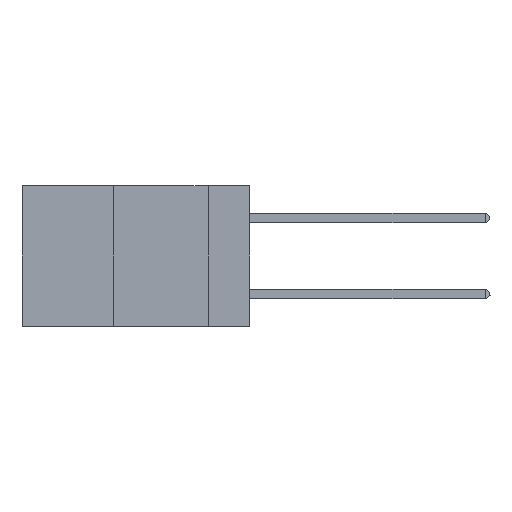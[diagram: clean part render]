
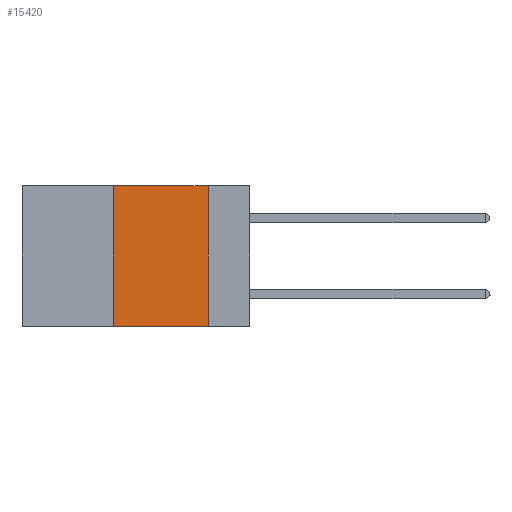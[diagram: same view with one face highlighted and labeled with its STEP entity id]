
A CAD part, left-side view. The second image highlights one B-rep face of the part: STEP entity #15420.
In plain terms, the highlighted planar face has unit normal (-1, 0, 0).
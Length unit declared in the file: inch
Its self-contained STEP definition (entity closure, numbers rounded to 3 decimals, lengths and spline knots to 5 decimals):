
#1288 = ORIENTED_EDGE ( 'NONE', *, *, #12858, .F. ) ;
#1420 = CARTESIAN_POINT ( 'NONE',  ( 0., 0.36, -0.37 ) ) ;
#1530 = VECTOR ( 'NONE', #26403, 39.37008 ) ;
#2300 = DIRECTION ( 'NONE',  ( 0., 0., -1. ) ) ;
#3197 = DIRECTION ( 'NONE',  ( 0., 0., 1. ) ) ;
#3232 = LINE ( 'NONE', #31575, #18596 ) ;
#4261 = ORIENTED_EDGE ( 'NONE', *, *, #20577, .T. ) ;
#4279 = LINE ( 'NONE', #28359, #14699 ) ;
#5063 = VERTEX_POINT ( 'NONE', #1420 ) ;
#5168 = CARTESIAN_POINT ( 'NONE',  ( 0., 0.11, 0. ) ) ;
#5804 = CARTESIAN_POINT ( 'NONE',  ( 0., 0.6, -0.37 ) ) ;
#7598 = ORIENTED_EDGE ( 'NONE', *, *, #31653, .F. ) ;
#11675 = ORIENTED_EDGE ( 'NONE', *, *, #27750, .F. ) ;
#12858 = EDGE_CURVE ( 'NONE', #24226, #24170, #3232, .T. ) ;
#13483 = DIRECTION ( 'NONE',  ( 0., 0., -1. ) ) ;
#13821 = AXIS2_PLACEMENT_3D ( 'NONE', #27410, #27300, #13483 ) ;
#14699 = VECTOR ( 'NONE', #3197, 39.37008 ) ;
#15420 = ADVANCED_FACE ( 'NONE', ( #19024 ), #35686, .F. ) ;
#15443 = VECTOR ( 'NONE', #2300, 39.37008 ) ;
#17627 = VERTEX_POINT ( 'NONE', #30947 ) ;
#18596 = VECTOR ( 'NONE', #23954, 39.37008 ) ;
#19024 = FACE_OUTER_BOUND ( 'NONE', #21722, .T. ) ;
#20577 = EDGE_CURVE ( 'NONE', #5063, #17627, #28182, .T. ) ;
#21722 = EDGE_LOOP ( 'NONE', ( #7598, #1288, #11675, #4261 ) ) ;
#23283 = LINE ( 'NONE', #30303, #15443 ) ;
#23954 = DIRECTION ( 'NONE',  ( 0., -1., 0. ) ) ;
#24170 = VERTEX_POINT ( 'NONE', #5168 ) ;
#24226 = VERTEX_POINT ( 'NONE', #30205 ) ;
#26403 = DIRECTION ( 'NONE',  ( 0., -1., 0. ) ) ;
#27300 = DIRECTION ( 'NONE',  ( 1., 0., 0. ) ) ;
#27410 = CARTESIAN_POINT ( 'NONE',  ( 0., 0.6, 0. ) ) ;
#27750 = EDGE_CURVE ( 'NONE', #5063, #24226, #4279, .T. ) ;
#28182 = LINE ( 'NONE', #5804, #1530 ) ;
#28359 = CARTESIAN_POINT ( 'NONE',  ( 0., 0.36, 0. ) ) ;
#30205 = CARTESIAN_POINT ( 'NONE',  ( 0., 0.36, 0. ) ) ;
#30303 = CARTESIAN_POINT ( 'NONE',  ( 0., 0.11, 0. ) ) ;
#30947 = CARTESIAN_POINT ( 'NONE',  ( 0., 0.11, -0.37 ) ) ;
#31575 = CARTESIAN_POINT ( 'NONE',  ( 0., 0.6, 0. ) ) ;
#31653 = EDGE_CURVE ( 'NONE', #24170, #17627, #23283, .T. ) ;
#35686 = PLANE ( 'NONE',  #13821 ) ;
